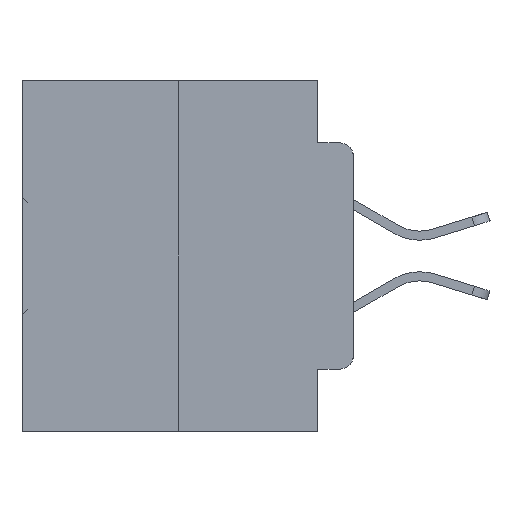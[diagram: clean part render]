
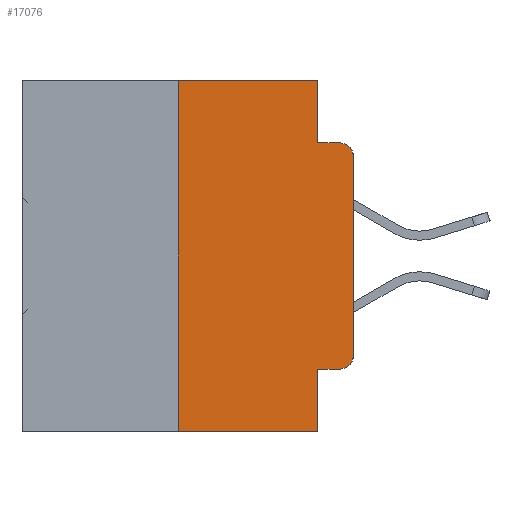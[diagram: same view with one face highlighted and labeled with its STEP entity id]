
A CAD part, left-side view. The second image highlights one B-rep face of the part: STEP entity #17076.
In plain terms, the highlighted planar face has unit normal (-1, 0, 0).
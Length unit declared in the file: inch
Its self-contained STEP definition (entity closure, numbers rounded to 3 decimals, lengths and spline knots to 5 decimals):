
#91 = DIRECTION ( 'NONE',  ( 0., 0., 1. ) ) ;
#277 = LINE ( 'NONE', #26358, #16721 ) ;
#496 = VECTOR ( 'NONE', #10353, 39.37008 ) ;
#1005 = VERTEX_POINT ( 'NONE', #24300 ) ;
#1055 = VECTOR ( 'NONE', #32070, 39.37008 ) ;
#2638 = DIRECTION ( 'NONE',  ( 0., -1., 0. ) ) ;
#2656 = VERTEX_POINT ( 'NONE', #20723 ) ;
#3117 = CARTESIAN_POINT ( 'NONE',  ( 0., 0.02, -0.3915 ) ) ;
#3321 = CARTESIAN_POINT ( 'NONE',  ( 0., 0.051, 0. ) ) ;
#3699 = CARTESIAN_POINT ( 'NONE',  ( 0., 0.051, -0.4115 ) ) ;
#4006 = EDGE_CURVE ( 'NONE', #2656, #11635, #9318, .T. ) ;
#5272 = DIRECTION ( 'NONE',  ( 0., -1., 0. ) ) ;
#5603 = ORIENTED_EDGE ( 'NONE', *, *, #26323, .T. ) ;
#5618 = ORIENTED_EDGE ( 'NONE', *, *, #26041, .T. ) ;
#5779 = VERTEX_POINT ( 'NONE', #10004 ) ;
#5805 = ORIENTED_EDGE ( 'NONE', *, *, #32157, .F. ) ;
#6882 = DIRECTION ( 'NONE',  ( 1., 0., 0. ) ) ;
#7883 = AXIS2_PLACEMENT_3D ( 'NONE', #22177, #6882, #33204 ) ;
#7991 = DIRECTION ( 'NONE',  ( 0., -1., 0. ) ) ;
#8976 = VECTOR ( 'NONE', #34328, 39.37008 ) ;
#9030 = EDGE_CURVE ( 'NONE', #20532, #19494, #30430, .T. ) ;
#9318 = LINE ( 'NONE', #17396, #8976 ) ;
#9886 = CARTESIAN_POINT ( 'NONE',  ( 0., 0.02, -0.0885 ) ) ;
#10004 = CARTESIAN_POINT ( 'NONE',  ( 0., 0.051, -0.4115 ) ) ;
#10353 = DIRECTION ( 'NONE',  ( 0., 0., 1. ) ) ;
#10912 = CARTESIAN_POINT ( 'NONE',  ( 0., 0.051, -0.0885 ) ) ;
#11635 = VERTEX_POINT ( 'NONE', #12417 ) ;
#12277 = AXIS2_PLACEMENT_3D ( 'NONE', #25217, #25973, #16982 ) ;
#12417 = CARTESIAN_POINT ( 'NONE',  ( 0., 0.051, -0.0885 ) ) ;
#14244 = VECTOR ( 'NONE', #7991, 39.37008 ) ;
#14580 = DIRECTION ( 'NONE',  ( -1., 0., 0. ) ) ;
#15124 = ORIENTED_EDGE ( 'NONE', *, *, #28553, .F. ) ;
#15160 = LINE ( 'NONE', #3321, #20254 ) ;
#15231 = EDGE_CURVE ( 'NONE', #1005, #20532, #16017, .T. ) ;
#15822 = ORIENTED_EDGE ( 'NONE', *, *, #9030, .T. ) ;
#15923 = EDGE_LOOP ( 'NONE', ( #15822, #16138, #15124, #16648, #27340, #5805, #5603, #24811, #5618, #21831 ) ) ;
#16017 = CIRCLE ( 'NONE', #36436, 0.02 ) ;
#16065 = CARTESIAN_POINT ( 'NONE',  ( 0., 0.25, -0.5 ) ) ;
#16078 = CARTESIAN_POINT ( 'NONE',  ( 0., 0.051, -0.5 ) ) ;
#16138 = ORIENTED_EDGE ( 'NONE', *, *, #23718, .T. ) ;
#16648 = ORIENTED_EDGE ( 'NONE', *, *, #4006, .F. ) ;
#16721 = VECTOR ( 'NONE', #91, 39.37008 ) ;
#16982 = DIRECTION ( 'NONE',  ( 0., 0., -1. ) ) ;
#17076 = ADVANCED_FACE ( 'NONE', ( #19175 ), #27818, .F. ) ;
#17396 = CARTESIAN_POINT ( 'NONE',  ( 0., 0.051, 0. ) ) ;
#19175 = FACE_OUTER_BOUND ( 'NONE', #15923, .T. ) ;
#19270 = VECTOR ( 'NONE', #5272, 39.37008 ) ;
#19494 = VERTEX_POINT ( 'NONE', #36868 ) ;
#20254 = VECTOR ( 'NONE', #32434, 39.37008 ) ;
#20532 = VERTEX_POINT ( 'NONE', #25988 ) ;
#20646 = LINE ( 'NONE', #32099, #19270 ) ;
#20723 = CARTESIAN_POINT ( 'NONE',  ( 0., 0.051, 0. ) ) ;
#21610 = CARTESIAN_POINT ( 'NONE',  ( 0., 0., 0. ) ) ;
#21831 = ORIENTED_EDGE ( 'NONE', *, *, #15231, .T. ) ;
#21895 = CARTESIAN_POINT ( 'NONE',  ( 0., 0.25, 0. ) ) ;
#22177 = CARTESIAN_POINT ( 'NONE',  ( 0., 0.473, 0. ) ) ;
#23151 = VERTEX_POINT ( 'NONE', #16078 ) ;
#23390 = DIRECTION ( 'NONE',  ( 0., 0., -1. ) ) ;
#23718 = EDGE_CURVE ( 'NONE', #19494, #36789, #26663, .T. ) ;
#24300 = CARTESIAN_POINT ( 'NONE',  ( 0., 0.02, -0.4115 ) ) ;
#24811 = ORIENTED_EDGE ( 'NONE', *, *, #26079, .F. ) ;
#25217 = CARTESIAN_POINT ( 'NONE',  ( 0., 0.02, -0.1085 ) ) ;
#25451 = LINE ( 'NONE', #31469, #14244 ) ;
#25973 = DIRECTION ( 'NONE',  ( -1., 0., 0. ) ) ;
#25988 = CARTESIAN_POINT ( 'NONE',  ( 0., 0., -0.3915 ) ) ;
#26041 = EDGE_CURVE ( 'NONE', #5779, #1005, #34892, .T. ) ;
#26079 = EDGE_CURVE ( 'NONE', #5779, #23151, #15160, .T. ) ;
#26159 = VERTEX_POINT ( 'NONE', #16065 ) ;
#26323 = EDGE_CURVE ( 'NONE', #26159, #23151, #25451, .T. ) ;
#26358 = CARTESIAN_POINT ( 'NONE',  ( 0., 0.25, 0. ) ) ;
#26663 = CIRCLE ( 'NONE', #12277, 0.02 ) ;
#27340 = ORIENTED_EDGE ( 'NONE', *, *, #29912, .F. ) ;
#27818 = PLANE ( 'NONE',  #7883 ) ;
#28553 = EDGE_CURVE ( 'NONE', #11635, #36789, #31184, .T. ) ;
#29912 = EDGE_CURVE ( 'NONE', #34254, #2656, #20646, .T. ) ;
#30430 = LINE ( 'NONE', #21610, #496 ) ;
#30585 = VECTOR ( 'NONE', #2638, 39.37008 ) ;
#31184 = LINE ( 'NONE', #10912, #30585 ) ;
#31469 = CARTESIAN_POINT ( 'NONE',  ( 0., 0.473, -0.5 ) ) ;
#32070 = DIRECTION ( 'NONE',  ( 0., -1., 0. ) ) ;
#32099 = CARTESIAN_POINT ( 'NONE',  ( 0., 0.473, 0. ) ) ;
#32157 = EDGE_CURVE ( 'NONE', #26159, #34254, #277, .T. ) ;
#32434 = DIRECTION ( 'NONE',  ( 0., 0., -1. ) ) ;
#33204 = DIRECTION ( 'NONE',  ( 0., 0., -1. ) ) ;
#34254 = VERTEX_POINT ( 'NONE', #21895 ) ;
#34328 = DIRECTION ( 'NONE',  ( 0., 0., -1. ) ) ;
#34892 = LINE ( 'NONE', #3699, #1055 ) ;
#36436 = AXIS2_PLACEMENT_3D ( 'NONE', #3117, #14580, #23390 ) ;
#36789 = VERTEX_POINT ( 'NONE', #9886 ) ;
#36868 = CARTESIAN_POINT ( 'NONE',  ( 0., 0., -0.1085 ) ) ;
